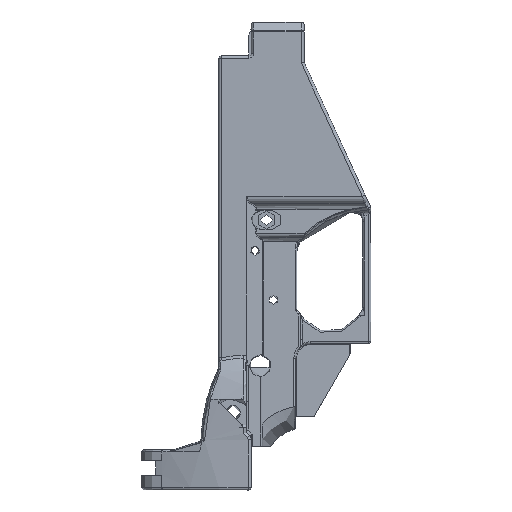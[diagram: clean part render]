
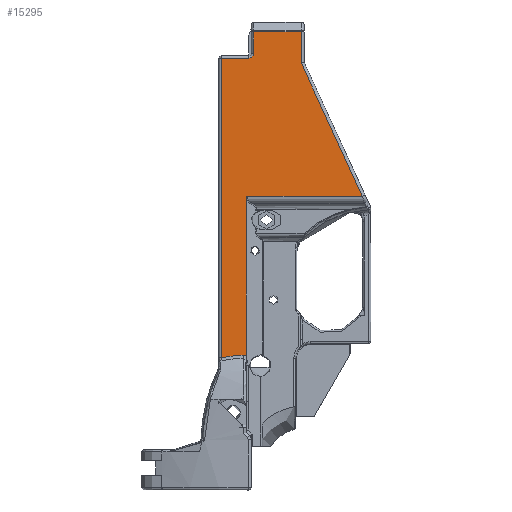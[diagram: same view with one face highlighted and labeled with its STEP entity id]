
A CAD part, left-side view. The second image highlights one B-rep face of the part: STEP entity #15295.
In plain terms, the highlighted planar face has unit normal (-1, 0, 0).
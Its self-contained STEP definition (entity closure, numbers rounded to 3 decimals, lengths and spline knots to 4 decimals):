
#219=ELLIPSE('',#16667,1.9201,1.636);
#399=PLANE('',#16665);
#1319=FACE_OUTER_BOUND('',#2274,.T.);
#2274=EDGE_LOOP('',(#12133,#12134,#12135,#12136,#12137,#12138,#12139,#12140,
#12141,#12142,#12143,#12144));
#3183=B_SPLINE_CURVE_WITH_KNOTS('',3,(#42398,#42399,#42400,#42401),
 .UNSPECIFIED.,.F.,.F.,(4,4),(-0.1434,0.),
 .UNSPECIFIED.);
#3184=B_SPLINE_CURVE_WITH_KNOTS('',3,(#42405,#42406,#42407,#42408,#42409,
#42410,#42411,#42412,#42413,#42414,#42415,#42416),.UNSPECIFIED.,.F.,.F.,
(4,2,2,2,2,4),(-0.117,-0.1147,-0.0798,
-0.057,-0.0072,0.),.UNSPECIFIED.);
#3818=CIRCLE('',#16666,0.08);
#4474=LINE('',#25050,#5242);
#4476=LINE('',#25081,#5244);
#4657=LINE('',#42350,#5425);
#4661=LINE('',#42388,#5429);
#4662=LINE('',#42392,#5430);
#4663=LINE('',#42394,#5431);
#4664=LINE('',#42403,#5432);
#4665=LINE('',#42417,#5433);
#5242=VECTOR('',#18787,0.3937);
#5244=VECTOR('',#18799,0.3937);
#5425=VECTOR('',#19654,0.3937);
#5429=VECTOR('',#19676,0.3937);
#5430=VECTOR('',#19679,0.3937);
#5431=VECTOR('',#19680,0.3937);
#5432=VECTOR('',#19683,1.6985);
#5433=VECTOR('',#19684,0.1181);
#6200=VERTEX_POINT('',#25047);
#6201=VERTEX_POINT('',#25049);
#6205=VERTEX_POINT('',#25079);
#6679=VERTEX_POINT('',#42348);
#6684=VERTEX_POINT('',#42387);
#6685=VERTEX_POINT('',#42389);
#6686=VERTEX_POINT('',#42391);
#6687=VERTEX_POINT('',#42393);
#6688=VERTEX_POINT('',#42395);
#6689=VERTEX_POINT('',#42397);
#6690=VERTEX_POINT('',#42402);
#6691=VERTEX_POINT('',#42404);
#7914=EDGE_CURVE('',#6200,#6201,#4474,.T.);
#7921=EDGE_CURVE('',#6205,#6200,#4476,.T.);
#8627=EDGE_CURVE('',#6679,#6205,#4657,.T.);
#8636=EDGE_CURVE('',#6684,#6679,#4661,.T.);
#8637=EDGE_CURVE('',#6685,#6684,#3818,.T.);
#8638=EDGE_CURVE('',#6686,#6685,#4662,.T.);
#8639=EDGE_CURVE('',#6687,#6686,#4663,.T.);
#8640=EDGE_CURVE('',#6688,#6687,#219,.T.);
#8641=EDGE_CURVE('',#6689,#6688,#3183,.T.);
#8642=EDGE_CURVE('',#6690,#6689,#4664,.T.);
#8643=EDGE_CURVE('',#6691,#6690,#3184,.T.);
#8644=EDGE_CURVE('',#6201,#6691,#4665,.T.);
#12133=ORIENTED_EDGE('',*,*,#7914,.F.);
#12134=ORIENTED_EDGE('',*,*,#7921,.F.);
#12135=ORIENTED_EDGE('',*,*,#8627,.F.);
#12136=ORIENTED_EDGE('',*,*,#8636,.F.);
#12137=ORIENTED_EDGE('',*,*,#8637,.F.);
#12138=ORIENTED_EDGE('',*,*,#8638,.F.);
#12139=ORIENTED_EDGE('',*,*,#8639,.F.);
#12140=ORIENTED_EDGE('',*,*,#8640,.F.);
#12141=ORIENTED_EDGE('',*,*,#8641,.F.);
#12142=ORIENTED_EDGE('',*,*,#8642,.F.);
#12143=ORIENTED_EDGE('',*,*,#8643,.F.);
#12144=ORIENTED_EDGE('',*,*,#8644,.F.);
#15295=ADVANCED_FACE('',(#1319),#399,.F.);
#16665=AXIS2_PLACEMENT_3D('',#42386,#19674,#19675);
#16666=AXIS2_PLACEMENT_3D('',#42390,#19677,#19678);
#16667=AXIS2_PLACEMENT_3D('',#42396,#19681,#19682);
#18787=DIRECTION('',(0.,-0.417,-0.909));
#18799=DIRECTION('',(0.,0.,-1.));
#19654=DIRECTION('',(0.,-1.,0.));
#19674=DIRECTION('center_axis',(1.,0.,0.));
#19675=DIRECTION('ref_axis',(0.,0.,
-1.));
#19676=DIRECTION('',(0.,0.,1.));
#19677=DIRECTION('center_axis',(-1.,0.,0.));
#19678=DIRECTION('ref_axis',(0.,-0.707,-0.707));
#19679=DIRECTION('',(0.,-1.,0.));
#19680=DIRECTION('',(0.,0.,1.));
#19681=DIRECTION('center_axis',(-1.,0.,0.));
#19682=DIRECTION('ref_axis',(0.,-0.984,-0.179));
#19683=DIRECTION('',(0.,0.,-1.));
#19684=DIRECTION('',(0.,1.,0.));
#25047=CARTESIAN_POINT('',(-0.731,-0.0727,2.8507));
#25049=CARTESIAN_POINT('',(-0.731,-1.118,0.5717));
#25050=CARTESIAN_POINT('',(-0.731,-1.4648,-0.1846));
#25079=CARTESIAN_POINT('',(-0.731,-0.0728,3.3816));
#25081=CARTESIAN_POINT('',(-0.731,-0.0727,-0.2092));
#42348=CARTESIAN_POINT('',(-0.731,0.7372,3.3816));
#42350=CARTESIAN_POINT('',(-0.731,0.7121,3.3816));
#42386=CARTESIAN_POINT('Origin',(-0.731,0.68,-3.6849));
#42387=CARTESIAN_POINT('',(-0.731,0.7373,3.0095));
#42388=CARTESIAN_POINT('',(-0.731,0.7373,-0.0118));
#42389=CARTESIAN_POINT('',(-0.731,0.8173,2.9295));
#42390=CARTESIAN_POINT('Origin',(-0.731,0.8173,3.0095));
#42391=CARTESIAN_POINT('',(-0.731,1.2902,2.9295));
#42392=CARTESIAN_POINT('',(-0.731,0.7441,2.9295));
#42393=CARTESIAN_POINT('',(-0.731,1.2902,-2.1813));
#42394=CARTESIAN_POINT('',(-0.731,1.2902,-3.1756));
#42395=CARTESIAN_POINT('',(-0.731,0.9158,-2.1342));
#42396=CARTESIAN_POINT('Origin',(-0.731,0.7244,-3.7785));
#42397=CARTESIAN_POINT('',(-0.731,0.8628,-2.151));
#42398=CARTESIAN_POINT('Ctrl Pts',(-0.731,0.8629,
-2.151));
#42399=CARTESIAN_POINT('Ctrl Pts',(-0.731,0.8784,
-2.1404));
#42400=CARTESIAN_POINT('Ctrl Pts',(-0.731,0.8969,
-2.1335));
#42401=CARTESIAN_POINT('Ctrl Pts',(-0.731,0.9158,
-2.1342));
#42402=CARTESIAN_POINT('',(-0.731,0.8628,0.5319));
#42403=CARTESIAN_POINT('',(-0.731,0.8628,-2.5001));
#42404=CARTESIAN_POINT('',(-0.731,0.8546,0.5717));
#42405=CARTESIAN_POINT('Ctrl Pts',(-0.731,0.8546,
0.5717));
#42406=CARTESIAN_POINT('Ctrl Pts',(-0.731,0.8546,
0.5716));
#42407=CARTESIAN_POINT('Ctrl Pts',(-0.731,0.8546,
0.5716));
#42408=CARTESIAN_POINT('Ctrl Pts',(-0.731,0.855,
0.5706));
#42409=CARTESIAN_POINT('Ctrl Pts',(-0.731,0.8564,
0.5674));
#42410=CARTESIAN_POINT('Ctrl Pts',(-0.731,0.8587,
0.5601));
#42411=CARTESIAN_POINT('Ctrl Pts',(-0.731,0.8595,
0.5572));
#42412=CARTESIAN_POINT('Ctrl Pts',(-0.731,0.8617,
0.5478));
#42413=CARTESIAN_POINT('Ctrl Pts',(-0.731,0.8626,
0.5413));
#42414=CARTESIAN_POINT('Ctrl Pts',(-0.731,0.8628,
0.5338));
#42415=CARTESIAN_POINT('Ctrl Pts',(-0.731,0.8628,
0.5329));
#42416=CARTESIAN_POINT('Ctrl Pts',(-0.731,0.8628,
0.5319));
#42417=CARTESIAN_POINT('',(-0.731,1.0895,0.5717));
